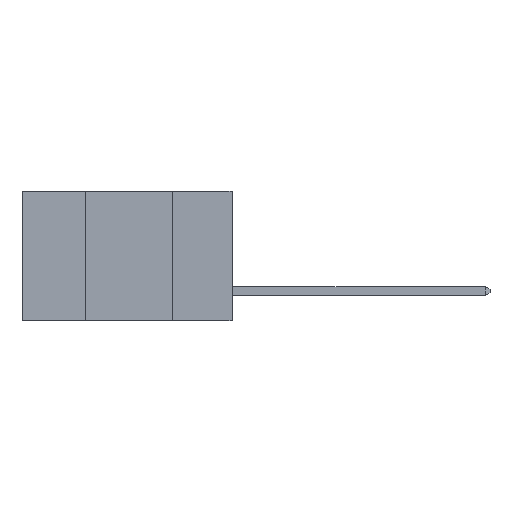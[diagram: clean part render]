
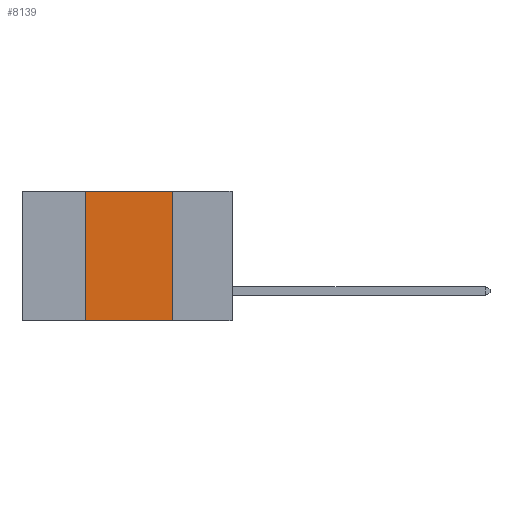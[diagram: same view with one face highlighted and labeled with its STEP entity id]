
A CAD part, left-side view. The second image highlights one B-rep face of the part: STEP entity #8139.
In plain terms, the highlighted planar face has unit normal (-1, 0, 0).
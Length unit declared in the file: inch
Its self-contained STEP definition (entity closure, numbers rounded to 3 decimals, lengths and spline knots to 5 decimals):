
#435 = EDGE_CURVE ( 'NONE', #1747, #6753, #1303, .T. ) ;
#979 = CARTESIAN_POINT ( 'NONE',  ( 0., 0.17, 0. ) ) ;
#1001 = VECTOR ( 'NONE', #9388, 39.37008 ) ;
#1303 = LINE ( 'NONE', #8324, #1001 ) ;
#1747 = VERTEX_POINT ( 'NONE', #979 ) ;
#1956 = CARTESIAN_POINT ( 'NONE',  ( 0., 0.6, 0. ) ) ;
#2905 = PLANE ( 'NONE',  #9588 ) ;
#2962 = EDGE_CURVE ( 'NONE', #7397, #1747, #7576, .T. ) ;
#3821 = DIRECTION ( 'NONE',  ( 1., 0., 0. ) ) ;
#4234 = LINE ( 'NONE', #9752, #6386 ) ;
#4335 = EDGE_LOOP ( 'NONE', ( #8308, #9596, #6868, #10179 ) ) ;
#4877 = VECTOR ( 'NONE', #11383, 39.37008 ) ;
#5261 = DIRECTION ( 'NONE',  ( 0., 0., 1. ) ) ;
#5392 = CARTESIAN_POINT ( 'NONE',  ( 0., 0.17, -0.37 ) ) ;
#5423 = EDGE_CURVE ( 'NONE', #10077, #7397, #4234, .T. ) ;
#5498 = VECTOR ( 'NONE', #6337, 39.37008 ) ;
#5624 = CARTESIAN_POINT ( 'NONE',  ( 0., 0.42, -0.37 ) ) ;
#5744 = FACE_OUTER_BOUND ( 'NONE', #4335, .T. ) ;
#6337 = DIRECTION ( 'NONE',  ( 0., -1., 0. ) ) ;
#6386 = VECTOR ( 'NONE', #5261, 39.37008 ) ;
#6753 = VERTEX_POINT ( 'NONE', #5392 ) ;
#6757 = EDGE_CURVE ( 'NONE', #10077, #6753, #8466, .T. ) ;
#6868 = ORIENTED_EDGE ( 'NONE', *, *, #5423, .F. ) ;
#7238 = CARTESIAN_POINT ( 'NONE',  ( 0., 0.42, 0. ) ) ;
#7397 = VERTEX_POINT ( 'NONE', #7238 ) ;
#7576 = LINE ( 'NONE', #10513, #4877 ) ;
#8139 = ADVANCED_FACE ( 'NONE', ( #5744 ), #2905, .F. ) ;
#8308 = ORIENTED_EDGE ( 'NONE', *, *, #435, .F. ) ;
#8324 = CARTESIAN_POINT ( 'NONE',  ( 0., 0.17, 0. ) ) ;
#8466 = LINE ( 'NONE', #10782, #5498 ) ;
#9388 = DIRECTION ( 'NONE',  ( 0., 0., -1. ) ) ;
#9588 = AXIS2_PLACEMENT_3D ( 'NONE', #1956, #3821, #10169 ) ;
#9596 = ORIENTED_EDGE ( 'NONE', *, *, #2962, .F. ) ;
#9752 = CARTESIAN_POINT ( 'NONE',  ( 0., 0.42, 0. ) ) ;
#10077 = VERTEX_POINT ( 'NONE', #5624 ) ;
#10169 = DIRECTION ( 'NONE',  ( 0., 0., -1. ) ) ;
#10179 = ORIENTED_EDGE ( 'NONE', *, *, #6757, .T. ) ;
#10513 = CARTESIAN_POINT ( 'NONE',  ( 0., 0.6, 0. ) ) ;
#10782 = CARTESIAN_POINT ( 'NONE',  ( 0., 0.6, -0.37 ) ) ;
#11383 = DIRECTION ( 'NONE',  ( 0., -1., 0. ) ) ;
